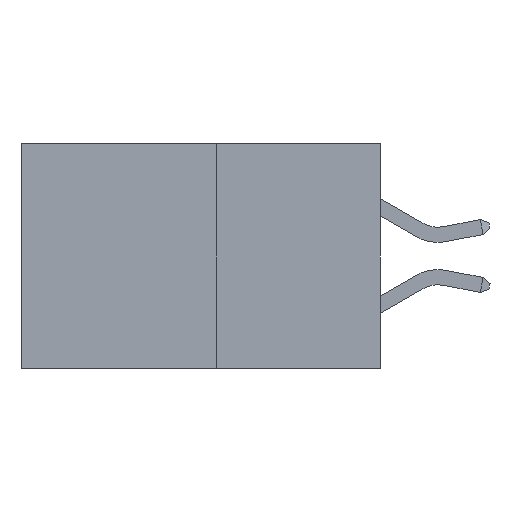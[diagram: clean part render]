
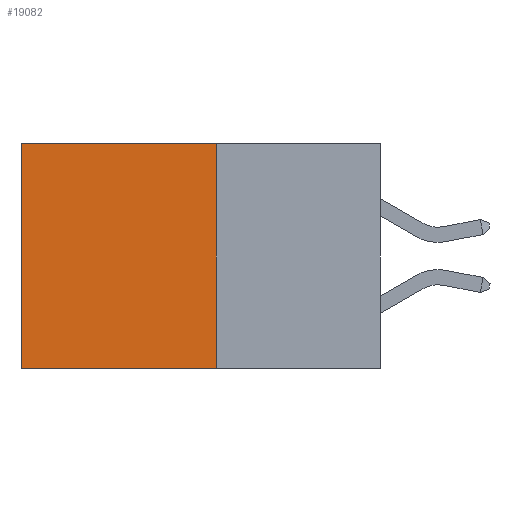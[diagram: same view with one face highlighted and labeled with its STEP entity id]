
A CAD part, left-side view. The second image highlights one B-rep face of the part: STEP entity #19082.
In plain terms, the highlighted planar face has unit normal (-1, 0, 0).
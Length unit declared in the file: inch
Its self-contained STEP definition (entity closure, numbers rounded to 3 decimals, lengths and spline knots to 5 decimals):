
#583 = ORIENTED_EDGE ( 'NONE', *, *, #675, .F. ) ;
#675 = EDGE_CURVE ( 'NONE', #21268, #4725, #21046, .T. ) ;
#976 = CARTESIAN_POINT ( 'NONE',  ( 0.277, 0.27, -0.37 ) ) ;
#1836 = EDGE_CURVE ( 'NONE', #4725, #10831, #16108, .T. ) ;
#2427 = CARTESIAN_POINT ( 'NONE',  ( 0.277, 0.27, -0.37 ) ) ;
#2750 = CARTESIAN_POINT ( 'NONE',  ( 0.277, 0.59, -0.37 ) ) ;
#3370 = CARTESIAN_POINT ( 'NONE',  ( 0.277, 0.59, -0.37 ) ) ;
#4578 = DIRECTION ( 'NONE',  ( 0., 0., -1. ) ) ;
#4693 = VECTOR ( 'NONE', #4578, 39.37008 ) ;
#4725 = VERTEX_POINT ( 'NONE', #6286 ) ;
#4791 = DIRECTION ( 'NONE',  ( 0., 1., 0. ) ) ;
#6028 = VECTOR ( 'NONE', #4791, 39.37008 ) ;
#6232 = VERTEX_POINT ( 'NONE', #15760 ) ;
#6286 = CARTESIAN_POINT ( 'NONE',  ( 0.277, 0.27, -0.37 ) ) ;
#7043 = ORIENTED_EDGE ( 'NONE', *, *, #1836, .F. ) ;
#7421 = DIRECTION ( 'NONE',  ( 0., 0., -1. ) ) ;
#7540 = VECTOR ( 'NONE', #7421, 39.37008 ) ;
#7726 = LINE ( 'NONE', #12153, #11874 ) ;
#8005 = FACE_OUTER_BOUND ( 'NONE', #9282, .T. ) ;
#8239 = PLANE ( 'NONE',  #21932 ) ;
#9282 = EDGE_LOOP ( 'NONE', ( #15390, #7043, #583, #12076 ) ) ;
#9507 = LINE ( 'NONE', #2750, #4693 ) ;
#10018 = DIRECTION ( 'NONE',  ( 0., 0., -1. ) ) ;
#10831 = VERTEX_POINT ( 'NONE', #3370 ) ;
#11035 = CARTESIAN_POINT ( 'NONE',  ( 0.277, 0.27, -0.37 ) ) ;
#11500 = EDGE_CURVE ( 'NONE', #21268, #6232, #7726, .T. ) ;
#11874 = VECTOR ( 'NONE', #17508, 39.37008 ) ;
#12021 = CARTESIAN_POINT ( 'NONE',  ( 0.277, 0.27, 0. ) ) ;
#12076 = ORIENTED_EDGE ( 'NONE', *, *, #11500, .T. ) ;
#12153 = CARTESIAN_POINT ( 'NONE',  ( 0.277, 0.27, 0. ) ) ;
#15390 = ORIENTED_EDGE ( 'NONE', *, *, #15976, .T. ) ;
#15760 = CARTESIAN_POINT ( 'NONE',  ( 0.277, 0.59, 0. ) ) ;
#15976 = EDGE_CURVE ( 'NONE', #6232, #10831, #9507, .T. ) ;
#16108 = LINE ( 'NONE', #2427, #6028 ) ;
#17508 = DIRECTION ( 'NONE',  ( 0., 1., 0. ) ) ;
#19082 = ADVANCED_FACE ( 'NONE', ( #8005 ), #8239, .F. ) ;
#20565 = DIRECTION ( 'NONE',  ( 1., 0., 0. ) ) ;
#21046 = LINE ( 'NONE', #11035, #7540 ) ;
#21268 = VERTEX_POINT ( 'NONE', #12021 ) ;
#21932 = AXIS2_PLACEMENT_3D ( 'NONE', #976, #20565, #10018 ) ;
